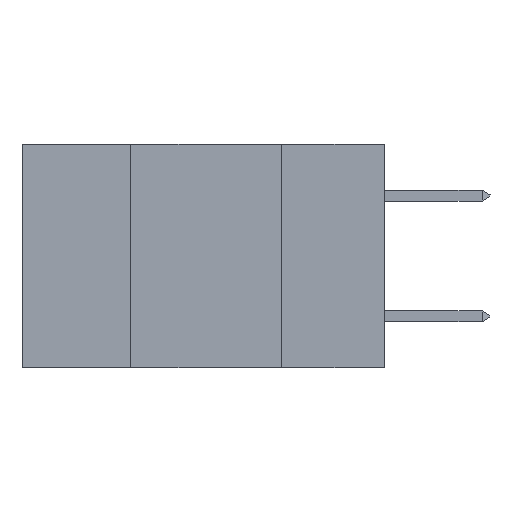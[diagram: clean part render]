
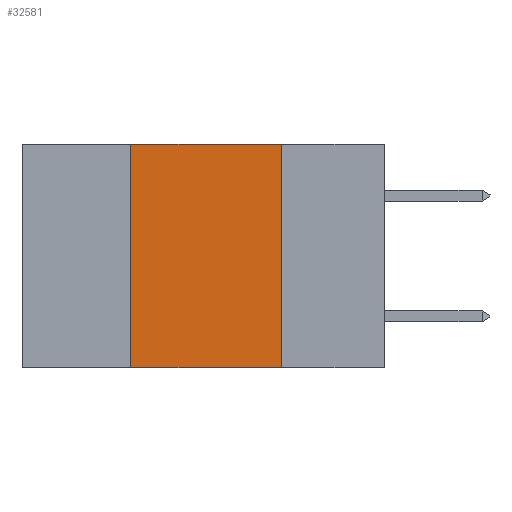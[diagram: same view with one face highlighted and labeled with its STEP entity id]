
A CAD part, left-side view. The second image highlights one B-rep face of the part: STEP entity #32581.
In plain terms, the highlighted planar face has unit normal (-1, 0, 0).
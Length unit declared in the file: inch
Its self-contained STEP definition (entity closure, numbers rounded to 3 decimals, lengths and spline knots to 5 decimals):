
#756 = VECTOR ( 'NONE', #15380, 39.37008 ) ;
#979 = CARTESIAN_POINT ( 'NONE',  ( 0., 0.17, 0. ) ) ;
#1701 = LINE ( 'NONE', #24564, #756 ) ;
#1889 = LINE ( 'NONE', #20237, #2803 ) ;
#2803 = VECTOR ( 'NONE', #26166, 39.37008 ) ;
#3143 = FACE_OUTER_BOUND ( 'NONE', #7982, .T. ) ;
#4706 = EDGE_CURVE ( 'NONE', #28451, #14608, #29412, .T. ) ;
#6897 = DIRECTION ( 'NONE',  ( 0., -1., 0. ) ) ;
#7982 = EDGE_LOOP ( 'NONE', ( #30369, #35417, #14997, #20760 ) ) ;
#8393 = PLANE ( 'NONE',  #32988 ) ;
#8668 = CARTESIAN_POINT ( 'NONE',  ( 0., 0.6, 0. ) ) ;
#13278 = LINE ( 'NONE', #25983, #35536 ) ;
#13350 = CARTESIAN_POINT ( 'NONE',  ( 0., 0.6, 0. ) ) ;
#13862 = EDGE_CURVE ( 'NONE', #25982, #28451, #1701, .T. ) ;
#14608 = VERTEX_POINT ( 'NONE', #979 ) ;
#14624 = VECTOR ( 'NONE', #6897, 39.37008 ) ;
#14997 = ORIENTED_EDGE ( 'NONE', *, *, #13862, .F. ) ;
#15380 = DIRECTION ( 'NONE',  ( 0., 0., 1. ) ) ;
#19425 = CARTESIAN_POINT ( 'NONE',  ( 0., 0.42, -0.37 ) ) ;
#20237 = CARTESIAN_POINT ( 'NONE',  ( 0., 0.6, -0.37 ) ) ;
#20760 = ORIENTED_EDGE ( 'NONE', *, *, #31100, .T. ) ;
#21843 = VERTEX_POINT ( 'NONE', #30577 ) ;
#22757 = DIRECTION ( 'NONE',  ( 0., 0., -1. ) ) ;
#24564 = CARTESIAN_POINT ( 'NONE',  ( 0., 0.42, 0. ) ) ;
#25982 = VERTEX_POINT ( 'NONE', #19425 ) ;
#25983 = CARTESIAN_POINT ( 'NONE',  ( 0., 0.17, 0. ) ) ;
#26118 = DIRECTION ( 'NONE',  ( 0., 0., -1. ) ) ;
#26166 = DIRECTION ( 'NONE',  ( 0., -1., 0. ) ) ;
#28451 = VERTEX_POINT ( 'NONE', #30951 ) ;
#29412 = LINE ( 'NONE', #13350, #14624 ) ;
#29602 = DIRECTION ( 'NONE',  ( 1., 0., 0. ) ) ;
#30369 = ORIENTED_EDGE ( 'NONE', *, *, #36143, .F. ) ;
#30577 = CARTESIAN_POINT ( 'NONE',  ( 0., 0.17, -0.37 ) ) ;
#30951 = CARTESIAN_POINT ( 'NONE',  ( 0., 0.42, 0. ) ) ;
#31100 = EDGE_CURVE ( 'NONE', #25982, #21843, #1889, .T. ) ;
#32581 = ADVANCED_FACE ( 'NONE', ( #3143 ), #8393, .F. ) ;
#32988 = AXIS2_PLACEMENT_3D ( 'NONE', #8668, #29602, #26118 ) ;
#35417 = ORIENTED_EDGE ( 'NONE', *, *, #4706, .F. ) ;
#35536 = VECTOR ( 'NONE', #22757, 39.37008 ) ;
#36143 = EDGE_CURVE ( 'NONE', #14608, #21843, #13278, .T. ) ;
